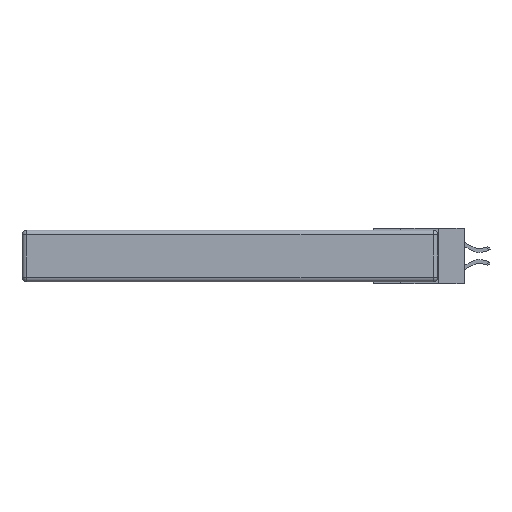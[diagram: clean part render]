
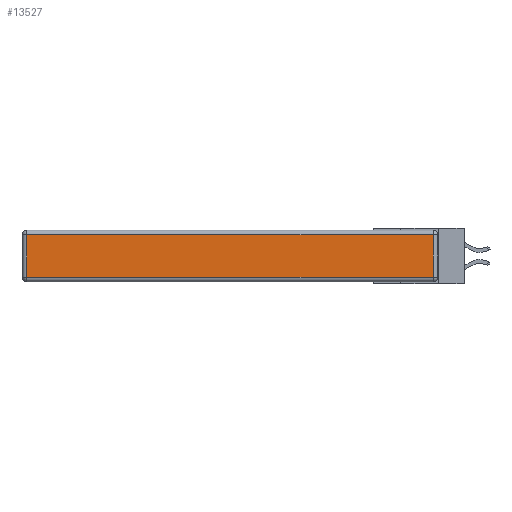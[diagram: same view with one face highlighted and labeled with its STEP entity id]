
A CAD part, left-side view. The second image highlights one B-rep face of the part: STEP entity #13527.
In plain terms, the highlighted planar face has unit normal (-1, 0, 0).
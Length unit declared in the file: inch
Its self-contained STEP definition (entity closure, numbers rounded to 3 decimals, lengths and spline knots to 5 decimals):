
#107 = DIRECTION ( 'NONE',  ( 0., 1., 0. ) ) ;
#472 = VECTOR ( 'NONE', #13751, 39.37008 ) ;
#595 = DIRECTION ( 'NONE',  ( 0., 0., 1. ) ) ;
#1024 = DIRECTION ( 'NONE',  ( 0., 0., 1. ) ) ;
#1308 = VERTEX_POINT ( 'NONE', #2485 ) ;
#1427 = ORIENTED_EDGE ( 'NONE', *, *, #10981, .T. ) ;
#1665 = EDGE_CURVE ( 'NONE', #12236, #11928, #4324, .T. ) ;
#2305 = ORIENTED_EDGE ( 'NONE', *, *, #14923, .T. ) ;
#2485 = CARTESIAN_POINT ( 'NONE',  ( 0., 2.72, -0.03 ) ) ;
#3345 = CARTESIAN_POINT ( 'NONE',  ( 0., 2.72, -0.343 ) ) ;
#3767 = ORIENTED_EDGE ( 'NONE', *, *, #1665, .T. ) ;
#4324 = LINE ( 'NONE', #10920, #8621 ) ;
#4420 = EDGE_LOOP ( 'NONE', ( #12735, #3767, #2305, #1427 ) ) ;
#5471 = DIRECTION ( 'NONE',  ( 0., -1., 0. ) ) ;
#6033 = LINE ( 'NONE', #3345, #472 ) ;
#6729 = CARTESIAN_POINT ( 'NONE',  ( 0., 0.03, -0.313 ) ) ;
#7203 = CARTESIAN_POINT ( 'NONE',  ( 0., 0.03, -0.03 ) ) ;
#8621 = VECTOR ( 'NONE', #595, 39.37008 ) ;
#9046 = PLANE ( 'NONE',  #11239 ) ;
#10211 = CARTESIAN_POINT ( 'NONE',  ( 0., 2.72, -0.313 ) ) ;
#10522 = LINE ( 'NONE', #15738, #11944 ) ;
#10757 = FACE_OUTER_BOUND ( 'NONE', #4420, .T. ) ;
#10920 = CARTESIAN_POINT ( 'NONE',  ( 0., 0.03, -0.343 ) ) ;
#10981 = EDGE_CURVE ( 'NONE', #1308, #12522, #6033, .T. ) ;
#11239 = AXIS2_PLACEMENT_3D ( 'NONE', #11427, #14120, #1024 ) ;
#11427 = CARTESIAN_POINT ( 'NONE',  ( 0., 0., -0.343 ) ) ;
#11922 = VECTOR ( 'NONE', #5471, 39.37008 ) ;
#11928 = VERTEX_POINT ( 'NONE', #7203 ) ;
#11944 = VECTOR ( 'NONE', #107, 39.37008 ) ;
#12236 = VERTEX_POINT ( 'NONE', #6729 ) ;
#12357 = LINE ( 'NONE', #13087, #11922 ) ;
#12522 = VERTEX_POINT ( 'NONE', #10211 ) ;
#12735 = ORIENTED_EDGE ( 'NONE', *, *, #15225, .T. ) ;
#13087 = CARTESIAN_POINT ( 'NONE',  ( 0., 0., -0.313 ) ) ;
#13527 = ADVANCED_FACE ( 'NONE', ( #10757 ), #9046, .T. ) ;
#13751 = DIRECTION ( 'NONE',  ( 0., 0., -1. ) ) ;
#14120 = DIRECTION ( 'NONE',  ( -1., 0., 0. ) ) ;
#14923 = EDGE_CURVE ( 'NONE', #11928, #1308, #10522, .T. ) ;
#15225 = EDGE_CURVE ( 'NONE', #12522, #12236, #12357, .T. ) ;
#15738 = CARTESIAN_POINT ( 'NONE',  ( 0., 2.75, -0.03 ) ) ;
